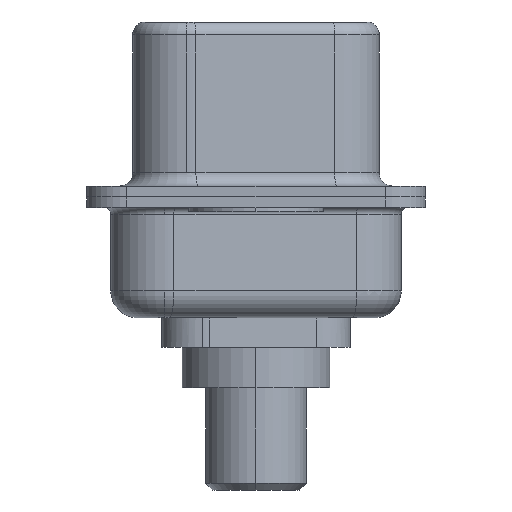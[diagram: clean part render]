
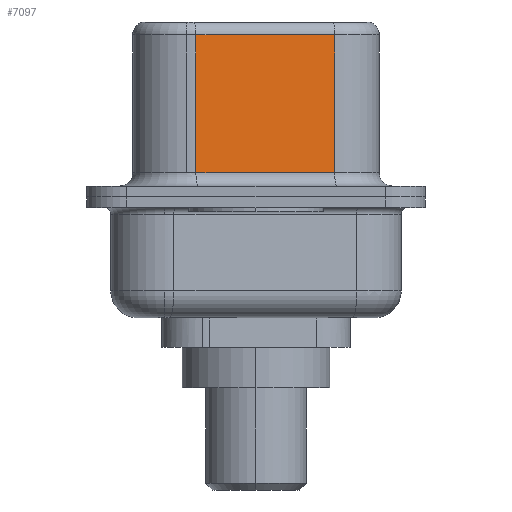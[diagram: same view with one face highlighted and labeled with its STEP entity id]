
A CAD part, left-side view. The second image highlights one B-rep face of the part: STEP entity #7097.
In plain terms, the highlighted planar face has unit normal (-0.985, -0.174, 0).
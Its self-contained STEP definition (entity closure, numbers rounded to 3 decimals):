
#322 = ORIENTED_EDGE ( 'NONE', *, *, #6292, .T. ) ;
#631 = LINE ( 'NONE', #8182, #9462 ) ;
#906 = DIRECTION ( 'NONE',  ( 0., 0., -1. ) ) ;
#1376 = ORIENTED_EDGE ( 'NONE', *, *, #4139, .F. ) ;
#1415 = VECTOR ( 'NONE', #906, 1000. ) ;
#1695 = LINE ( 'NONE', #1872, #1415 ) ;
#1872 = CARTESIAN_POINT ( 'NONE',  ( 3.655, 2.233, 6.52 ) ) ;
#1920 = VERTEX_POINT ( 'NONE', #5151 ) ;
#2359 = DIRECTION ( 'NONE',  ( 0.174, -0.985, 0. ) ) ;
#2537 = CARTESIAN_POINT ( 'NONE',  ( 3.655, 2.233, 0.9 ) ) ;
#3548 = CARTESIAN_POINT ( 'NONE',  ( 4.565, -2.927, 0.9 ) ) ;
#3840 = LINE ( 'NONE', #7983, #6142 ) ;
#4139 = EDGE_CURVE ( 'NONE', #1920, #7622, #3840, .T. ) ;
#4270 = VERTEX_POINT ( 'NONE', #8065 ) ;
#5096 = ORIENTED_EDGE ( 'NONE', *, *, #6814, .T. ) ;
#5151 = CARTESIAN_POINT ( 'NONE',  ( 4.565, -2.927, 6.02 ) ) ;
#5264 = FACE_OUTER_BOUND ( 'NONE', #7369, .T. ) ;
#5342 = DIRECTION ( 'NONE',  ( -0.174, 0.985, 0. ) ) ;
#6142 = VECTOR ( 'NONE', #6718, 1000. ) ;
#6292 = EDGE_CURVE ( 'NONE', #10303, #7622, #8697, .T. ) ;
#6342 = PLANE ( 'NONE',  #10890 ) ;
#6718 = DIRECTION ( 'NONE',  ( 0., 0., -1. ) ) ;
#6814 = EDGE_CURVE ( 'NONE', #1920, #4270, #631, .T. ) ;
#7097 = ADVANCED_FACE ( 'NONE', ( #5264 ), #6342, .F. ) ;
#7252 = VECTOR ( 'NONE', #2359, 1000. ) ;
#7369 = EDGE_LOOP ( 'NONE', ( #1376, #5096, #8944, #322 ) ) ;
#7622 = VERTEX_POINT ( 'NONE', #9117 ) ;
#7983 = CARTESIAN_POINT ( 'NONE',  ( 4.565, -2.927, 6.52 ) ) ;
#8012 = EDGE_CURVE ( 'NONE', #4270, #10303, #1695, .T. ) ;
#8065 = CARTESIAN_POINT ( 'NONE',  ( 3.655, 2.233, 6.02 ) ) ;
#8182 = CARTESIAN_POINT ( 'NONE',  ( 4.565, -2.927, 6.02 ) ) ;
#8697 = LINE ( 'NONE', #3548, #7252 ) ;
#8944 = ORIENTED_EDGE ( 'NONE', *, *, #8012, .T. ) ;
#9117 = CARTESIAN_POINT ( 'NONE',  ( 4.565, -2.927, 0.9 ) ) ;
#9279 = CARTESIAN_POINT ( 'NONE',  ( 4.565, -2.927, 6.52 ) ) ;
#9462 = VECTOR ( 'NONE', #5342, 1000. ) ;
#10303 = VERTEX_POINT ( 'NONE', #2537 ) ;
#10890 = AXIS2_PLACEMENT_3D ( 'NONE', #9279, #10902, #10916 ) ;
#10902 = DIRECTION ( 'NONE',  ( 0.985, 0.174, 0. ) ) ;
#10916 = DIRECTION ( 'NONE',  ( -0.174, 0.985, 0. ) ) ;
